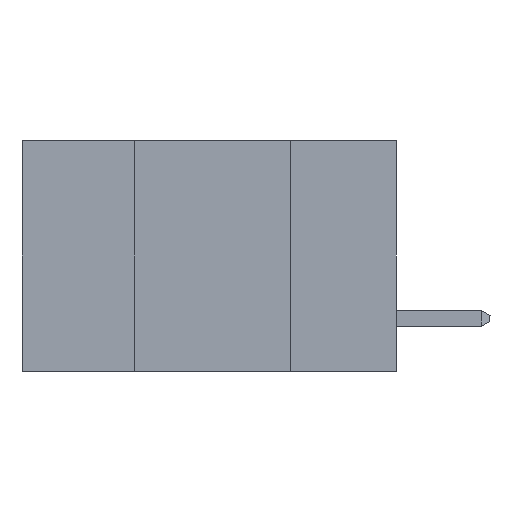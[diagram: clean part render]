
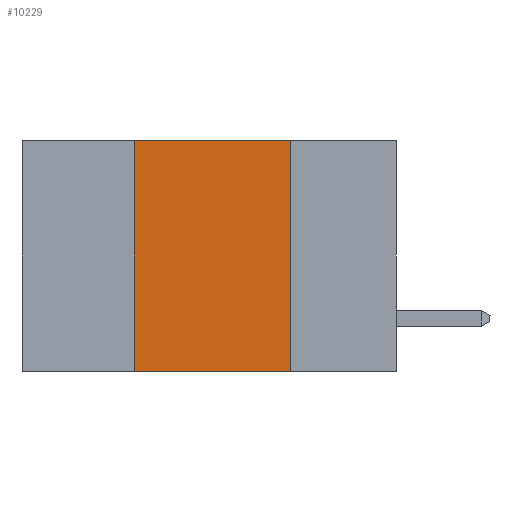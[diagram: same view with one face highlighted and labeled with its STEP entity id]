
A CAD part, left-side view. The second image highlights one B-rep face of the part: STEP entity #10229.
In plain terms, the highlighted planar face has unit normal (-1, 0, 0).
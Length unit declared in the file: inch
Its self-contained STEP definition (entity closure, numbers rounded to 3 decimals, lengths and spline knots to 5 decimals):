
#615 = CARTESIAN_POINT ( 'NONE',  ( 0., 0.42, -0.37 ) ) ;
#1449 = CARTESIAN_POINT ( 'NONE',  ( 0., 0.17, 0. ) ) ;
#2302 = ORIENTED_EDGE ( 'NONE', *, *, #21179, .F. ) ;
#2351 = CARTESIAN_POINT ( 'NONE',  ( 0., 0.6, 0. ) ) ;
#2979 = VECTOR ( 'NONE', #17307, 39.37008 ) ;
#4314 = EDGE_CURVE ( 'NONE', #4553, #10693, #21671, .T. ) ;
#4553 = VERTEX_POINT ( 'NONE', #11086 ) ;
#4993 = DIRECTION ( 'NONE',  ( 0., -1., 0. ) ) ;
#5541 = CARTESIAN_POINT ( 'NONE',  ( 0., 0.6, 0. ) ) ;
#6545 = CARTESIAN_POINT ( 'NONE',  ( 0., 0.6, -0.37 ) ) ;
#6561 = EDGE_CURVE ( 'NONE', #18055, #10693, #16834, .T. ) ;
#7243 = ORIENTED_EDGE ( 'NONE', *, *, #6561, .F. ) ;
#7527 = DIRECTION ( 'NONE',  ( 0., 0., -1. ) ) ;
#7836 = EDGE_LOOP ( 'NONE', ( #7243, #2302, #12617, #7973 ) ) ;
#7973 = ORIENTED_EDGE ( 'NONE', *, *, #4314, .T. ) ;
#8377 = DIRECTION ( 'NONE',  ( 0., 0., -1. ) ) ;
#9192 = LINE ( 'NONE', #615, #2979 ) ;
#9281 = VECTOR ( 'NONE', #4993, 39.37008 ) ;
#9578 = LINE ( 'NONE', #2351, #20084 ) ;
#9582 = AXIS2_PLACEMENT_3D ( 'NONE', #5541, #10862, #7527 ) ;
#10229 = ADVANCED_FACE ( 'NONE', ( #13968 ), #20651, .F. ) ;
#10693 = VERTEX_POINT ( 'NONE', #17924 ) ;
#10862 = DIRECTION ( 'NONE',  ( 1., 0., 0. ) ) ;
#11086 = CARTESIAN_POINT ( 'NONE',  ( 0., 0.42, -0.37 ) ) ;
#12132 = CARTESIAN_POINT ( 'NONE',  ( 0., 0.42, 0. ) ) ;
#12617 = ORIENTED_EDGE ( 'NONE', *, *, #18715, .F. ) ;
#13204 = VERTEX_POINT ( 'NONE', #12132 ) ;
#13968 = FACE_OUTER_BOUND ( 'NONE', #7836, .T. ) ;
#16267 = VECTOR ( 'NONE', #8377, 39.37008 ) ;
#16834 = LINE ( 'NONE', #20163, #16267 ) ;
#17307 = DIRECTION ( 'NONE',  ( 0., 0., 1. ) ) ;
#17804 = DIRECTION ( 'NONE',  ( 0., -1., 0. ) ) ;
#17924 = CARTESIAN_POINT ( 'NONE',  ( 0., 0.17, -0.37 ) ) ;
#18055 = VERTEX_POINT ( 'NONE', #1449 ) ;
#18715 = EDGE_CURVE ( 'NONE', #4553, #13204, #9192, .T. ) ;
#20084 = VECTOR ( 'NONE', #17804, 39.37008 ) ;
#20163 = CARTESIAN_POINT ( 'NONE',  ( 0., 0.17, -0.37 ) ) ;
#20651 = PLANE ( 'NONE',  #9582 ) ;
#21179 = EDGE_CURVE ( 'NONE', #13204, #18055, #9578, .T. ) ;
#21671 = LINE ( 'NONE', #6545, #9281 ) ;
